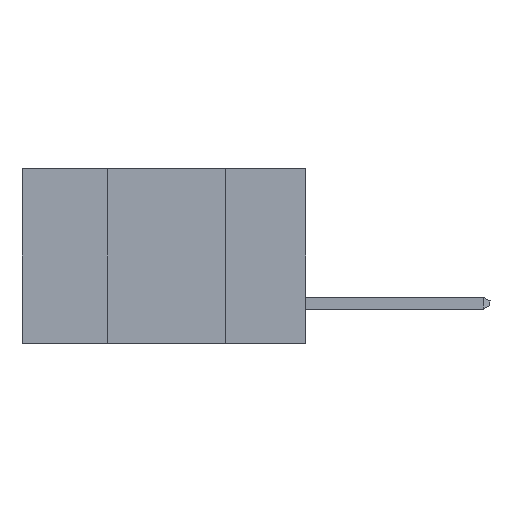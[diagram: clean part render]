
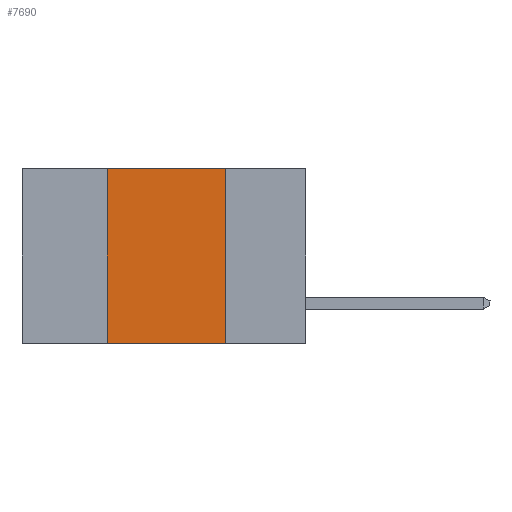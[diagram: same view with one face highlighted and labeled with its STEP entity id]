
A CAD part, left-side view. The second image highlights one B-rep face of the part: STEP entity #7690.
In plain terms, the highlighted planar face has unit normal (-1, 0, 0).
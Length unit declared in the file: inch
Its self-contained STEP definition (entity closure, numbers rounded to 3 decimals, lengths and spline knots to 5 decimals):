
#535 = DIRECTION ( 'NONE',  ( 0., 0., -1. ) ) ;
#900 = DIRECTION ( 'NONE',  ( 0., 0., 1. ) ) ;
#1819 = CARTESIAN_POINT ( 'NONE',  ( 0., 0.42, 0. ) ) ;
#2190 = VERTEX_POINT ( 'NONE', #1819 ) ;
#3314 = EDGE_CURVE ( 'NONE', #19428, #11197, #7380, .T. ) ;
#4666 = CARTESIAN_POINT ( 'NONE',  ( 0., 0.42, -0.37 ) ) ;
#4764 = ORIENTED_EDGE ( 'NONE', *, *, #9049, .F. ) ;
#4882 = CARTESIAN_POINT ( 'NONE',  ( 0., 0.6, -0.37 ) ) ;
#5473 = AXIS2_PLACEMENT_3D ( 'NONE', #17907, #8344, #535 ) ;
#5518 = VECTOR ( 'NONE', #12563, 39.37008 ) ;
#6944 = LINE ( 'NONE', #4666, #22813 ) ;
#7051 = VERTEX_POINT ( 'NONE', #22426 ) ;
#7252 = DIRECTION ( 'NONE',  ( 0., 0., -1. ) ) ;
#7380 = LINE ( 'NONE', #9393, #21450 ) ;
#7690 = ADVANCED_FACE ( 'NONE', ( #8222 ), #13520, .F. ) ;
#7973 = EDGE_CURVE ( 'NONE', #2190, #19428, #16772, .T. ) ;
#8222 = FACE_OUTER_BOUND ( 'NONE', #9254, .T. ) ;
#8344 = DIRECTION ( 'NONE',  ( 1., 0., 0. ) ) ;
#8707 = ORIENTED_EDGE ( 'NONE', *, *, #15043, .T. ) ;
#9049 = EDGE_CURVE ( 'NONE', #7051, #2190, #6944, .T. ) ;
#9254 = EDGE_LOOP ( 'NONE', ( #22580, #17725, #4764, #8707 ) ) ;
#9393 = CARTESIAN_POINT ( 'NONE',  ( 0., 0.17, -0.37 ) ) ;
#10174 = CARTESIAN_POINT ( 'NONE',  ( 0., 0.17, -0.37 ) ) ;
#11197 = VERTEX_POINT ( 'NONE', #10174 ) ;
#12197 = LINE ( 'NONE', #4882, #5518 ) ;
#12563 = DIRECTION ( 'NONE',  ( 0., -1., 0. ) ) ;
#12731 = VECTOR ( 'NONE', #20659, 39.37008 ) ;
#13520 = PLANE ( 'NONE',  #5473 ) ;
#15043 = EDGE_CURVE ( 'NONE', #7051, #11197, #12197, .T. ) ;
#16772 = LINE ( 'NONE', #24430, #12731 ) ;
#16834 = CARTESIAN_POINT ( 'NONE',  ( 0., 0.17, 0. ) ) ;
#17725 = ORIENTED_EDGE ( 'NONE', *, *, #7973, .F. ) ;
#17907 = CARTESIAN_POINT ( 'NONE',  ( 0., 0.6, 0. ) ) ;
#19428 = VERTEX_POINT ( 'NONE', #16834 ) ;
#20659 = DIRECTION ( 'NONE',  ( 0., -1., 0. ) ) ;
#21450 = VECTOR ( 'NONE', #7252, 39.37008 ) ;
#22426 = CARTESIAN_POINT ( 'NONE',  ( 0., 0.42, -0.37 ) ) ;
#22580 = ORIENTED_EDGE ( 'NONE', *, *, #3314, .F. ) ;
#22813 = VECTOR ( 'NONE', #900, 39.37008 ) ;
#24430 = CARTESIAN_POINT ( 'NONE',  ( 0., 0.6, 0. ) ) ;
